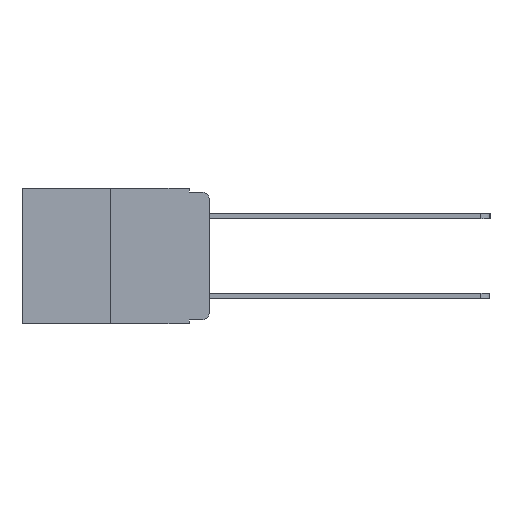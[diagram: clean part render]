
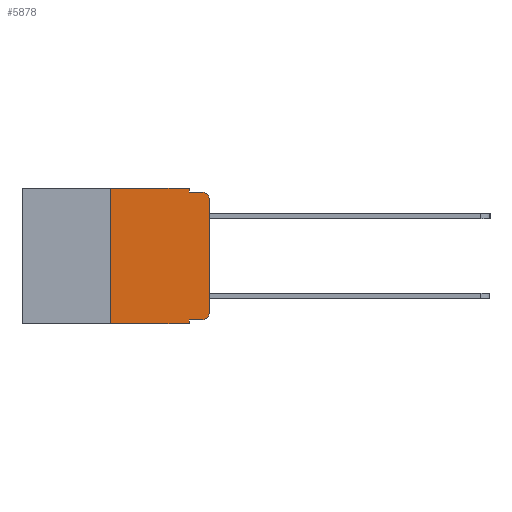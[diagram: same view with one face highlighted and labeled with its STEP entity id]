
A CAD part, left-side view. The second image highlights one B-rep face of the part: STEP entity #5878.
In plain terms, the highlighted planar face has unit normal (-1, 0, 0).
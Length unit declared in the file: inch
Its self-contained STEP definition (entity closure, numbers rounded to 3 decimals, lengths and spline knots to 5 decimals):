
#4 = CARTESIAN_POINT ( 'NONE',  ( 0., 0.051, 0. ) ) ;
#45 = VECTOR ( 'NONE', #7129, 39.37008 ) ;
#57 = VECTOR ( 'NONE', #3117, 39.37008 ) ;
#192 = VECTOR ( 'NONE', #5947, 39.37008 ) ;
#401 = CARTESIAN_POINT ( 'NONE',  ( 0., 0., -0.313 ) ) ;
#476 = VERTEX_POINT ( 'NONE', #4941 ) ;
#734 = LINE ( 'NONE', #6825, #10005 ) ;
#1016 = DIRECTION ( 'NONE',  ( 0., 0., -1. ) ) ;
#1359 = EDGE_LOOP ( 'NONE', ( #7455, #7375, #7122, #4926, #4801, #4699, #4445, #4344, #3958, #3895 ) ) ;
#1370 = LINE ( 'NONE', #8206, #192 ) ;
#1578 = VECTOR ( 'NONE', #3670, 39.37008 ) ;
#1687 = EDGE_CURVE ( 'NONE', #5625, #11541, #10488, .T. ) ;
#2387 = VERTEX_POINT ( 'NONE', #10547 ) ;
#2547 = LINE ( 'NONE', #7093, #57 ) ;
#2647 = EDGE_CURVE ( 'NONE', #10042, #5649, #5870, .T. ) ;
#2884 = VERTEX_POINT ( 'NONE', #7454 ) ;
#3117 = DIRECTION ( 'NONE',  ( 0., -1., 0. ) ) ;
#3305 = CARTESIAN_POINT ( 'NONE',  ( 0., 0.02, -0.01 ) ) ;
#3567 = CARTESIAN_POINT ( 'NONE',  ( 0., 0.02, -0.03 ) ) ;
#3670 = DIRECTION ( 'NONE',  ( 0., -1., 0. ) ) ;
#3715 = CARTESIAN_POINT ( 'NONE',  ( 0., 0.051, 0. ) ) ;
#3895 = ORIENTED_EDGE ( 'NONE', *, *, #2647, .T. ) ;
#3945 = EDGE_CURVE ( 'NONE', #5649, #6540, #6598, .T. ) ;
#3958 = ORIENTED_EDGE ( 'NONE', *, *, #5042, .T. ) ;
#4144 = EDGE_CURVE ( 'NONE', #5625, #2387, #2547, .T. ) ;
#4234 = CARTESIAN_POINT ( 'NONE',  ( 0., 0.25, 0. ) ) ;
#4344 = ORIENTED_EDGE ( 'NONE', *, *, #5798, .F. ) ;
#4436 = DIRECTION ( 'NONE',  ( 0., 0., -1. ) ) ;
#4445 = ORIENTED_EDGE ( 'NONE', *, *, #4144, .T. ) ;
#4699 = ORIENTED_EDGE ( 'NONE', *, *, #1687, .F. ) ;
#4746 = EDGE_CURVE ( 'NONE', #7462, #476, #7869, .T. ) ;
#4764 = VERTEX_POINT ( 'NONE', #3305 ) ;
#4801 = ORIENTED_EDGE ( 'NONE', *, *, #7760, .F. ) ;
#4856 = CARTESIAN_POINT ( 'NONE',  ( 0., 0., -0.03 ) ) ;
#4926 = ORIENTED_EDGE ( 'NONE', *, *, #4746, .F. ) ;
#4941 = CARTESIAN_POINT ( 'NONE',  ( 0., 0.051, -0.01 ) ) ;
#5042 = EDGE_CURVE ( 'NONE', #2884, #10042, #1370, .T. ) ;
#5228 = DIRECTION ( 'NONE',  ( 0., 0., -1. ) ) ;
#5274 = CARTESIAN_POINT ( 'NONE',  ( 0., 0.25, 0. ) ) ;
#5625 = VERTEX_POINT ( 'NONE', #6244 ) ;
#5649 = VERTEX_POINT ( 'NONE', #401 ) ;
#5798 = EDGE_CURVE ( 'NONE', #2884, #2387, #7300, .T. ) ;
#5870 = CIRCLE ( 'NONE', #11266, 0.02 ) ;
#5878 = ADVANCED_FACE ( 'NONE', ( #8296 ), #9944, .F. ) ;
#5947 = DIRECTION ( 'NONE',  ( 0., -1., 0. ) ) ;
#5976 = DIRECTION ( 'NONE',  ( 0., 0., 1. ) ) ;
#6111 = CARTESIAN_POINT ( 'NONE',  ( 0., 0.02, -0.333 ) ) ;
#6168 = AXIS2_PLACEMENT_3D ( 'NONE', #8214, #6398, #1016 ) ;
#6244 = CARTESIAN_POINT ( 'NONE',  ( 0., 0.25, -0.343 ) ) ;
#6398 = DIRECTION ( 'NONE',  ( 1., 0., 0. ) ) ;
#6540 = VERTEX_POINT ( 'NONE', #4856 ) ;
#6598 = LINE ( 'NONE', #8866, #9269 ) ;
#6825 = CARTESIAN_POINT ( 'NONE',  ( 0., 0.473, 0. ) ) ;
#6994 = VECTOR ( 'NONE', #5228, 39.37008 ) ;
#7083 = CARTESIAN_POINT ( 'NONE',  ( 0., 0.051, 0. ) ) ;
#7093 = CARTESIAN_POINT ( 'NONE',  ( 0., 0.473, -0.343 ) ) ;
#7122 = ORIENTED_EDGE ( 'NONE', *, *, #7457, .F. ) ;
#7129 = DIRECTION ( 'NONE',  ( 0., 0., -1. ) ) ;
#7300 = LINE ( 'NONE', #7083, #6994 ) ;
#7375 = ORIENTED_EDGE ( 'NONE', *, *, #10090, .T. ) ;
#7454 = CARTESIAN_POINT ( 'NONE',  ( 0., 0.051, -0.333 ) ) ;
#7455 = ORIENTED_EDGE ( 'NONE', *, *, #3945, .T. ) ;
#7457 = EDGE_CURVE ( 'NONE', #476, #4764, #11012, .T. ) ;
#7462 = VERTEX_POINT ( 'NONE', #4 ) ;
#7760 = EDGE_CURVE ( 'NONE', #11541, #7462, #734, .T. ) ;
#7869 = LINE ( 'NONE', #3715, #45 ) ;
#8114 = DIRECTION ( 'NONE',  ( 0., 0., 1. ) ) ;
#8206 = CARTESIAN_POINT ( 'NONE',  ( 0., 0.051, -0.333 ) ) ;
#8214 = CARTESIAN_POINT ( 'NONE',  ( 0., 0.473, 0. ) ) ;
#8228 = VECTOR ( 'NONE', #5976, 39.37008 ) ;
#8296 = FACE_OUTER_BOUND ( 'NONE', #1359, .T. ) ;
#8386 = AXIS2_PLACEMENT_3D ( 'NONE', #3567, #9800, #4436 ) ;
#8651 = DIRECTION ( 'NONE',  ( 0., -1., 0. ) ) ;
#8773 = CARTESIAN_POINT ( 'NONE',  ( 0., 0.02, -0.313 ) ) ;
#8866 = CARTESIAN_POINT ( 'NONE',  ( 0., 0., 0. ) ) ;
#9269 = VECTOR ( 'NONE', #8114, 39.37008 ) ;
#9729 = CIRCLE ( 'NONE', #8386, 0.02 ) ;
#9800 = DIRECTION ( 'NONE',  ( -1., 0., 0. ) ) ;
#9910 = CARTESIAN_POINT ( 'NONE',  ( 0., 0.051, -0.01 ) ) ;
#9944 = PLANE ( 'NONE',  #6168 ) ;
#10005 = VECTOR ( 'NONE', #8651, 39.37008 ) ;
#10042 = VERTEX_POINT ( 'NONE', #6111 ) ;
#10090 = EDGE_CURVE ( 'NONE', #6540, #4764, #9729, .T. ) ;
#10408 = DIRECTION ( 'NONE',  ( 0., 0., -1. ) ) ;
#10488 = LINE ( 'NONE', #5274, #8228 ) ;
#10496 = DIRECTION ( 'NONE',  ( -1., 0., 0. ) ) ;
#10547 = CARTESIAN_POINT ( 'NONE',  ( 0., 0.051, -0.343 ) ) ;
#11012 = LINE ( 'NONE', #9910, #1578 ) ;
#11266 = AXIS2_PLACEMENT_3D ( 'NONE', #8773, #10496, #10408 ) ;
#11541 = VERTEX_POINT ( 'NONE', #4234 ) ;
